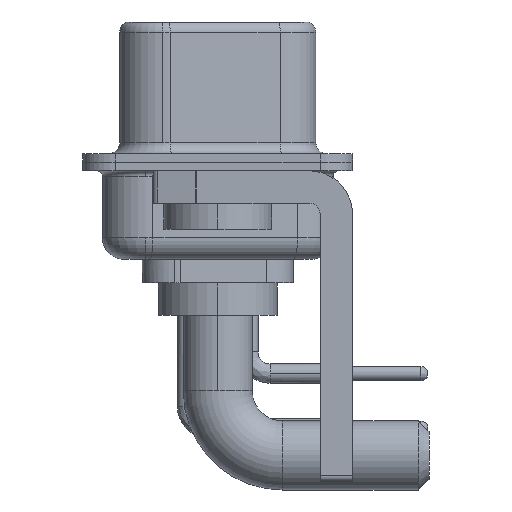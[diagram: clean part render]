
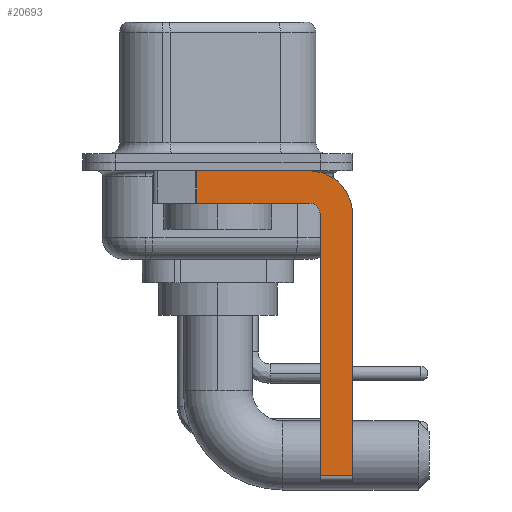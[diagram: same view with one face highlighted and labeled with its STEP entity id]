
A CAD part, left-side view. The second image highlights one B-rep face of the part: STEP entity #20693.
In plain terms, the highlighted planar face has unit normal (-1, 0, 0).
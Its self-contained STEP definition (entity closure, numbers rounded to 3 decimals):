
#100 = CARTESIAN_POINT ( 'NONE',  ( -2.9, -6.25, -2.4 ) ) ;
#116 = VECTOR ( 'NONE', #11203, 1000. ) ;
#220 = CARTESIAN_POINT ( 'NONE',  ( -2.9, 0.978, -1.9 ) ) ;
#757 = AXIS2_PLACEMENT_3D ( 'NONE', #5977, #12629, #12404 ) ;
#1545 = DIRECTION ( 'NONE',  ( 0., 0., -1. ) ) ;
#1931 = ORIENTED_EDGE ( 'NONE', *, *, #10886, .T. ) ;
#2019 = DIRECTION ( 'NONE',  ( 1., 0., 0. ) ) ;
#2078 = ORIENTED_EDGE ( 'NONE', *, *, #13336, .F. ) ;
#2173 = VECTOR ( 'NONE', #6767, 1000. ) ;
#2794 = VERTEX_POINT ( 'NONE', #19829 ) ;
#2855 = CIRCLE ( 'NONE', #9224, 2. ) ;
#3239 = CARTESIAN_POINT ( 'NONE',  ( -2.9, -4.25, -14.55 ) ) ;
#3648 = DIRECTION ( 'NONE',  ( 0., 0., -1. ) ) ;
#3952 = VERTEX_POINT ( 'NONE', #18066 ) ;
#4442 = AXIS2_PLACEMENT_3D ( 'NONE', #19038, #2019, #8884 ) ;
#4966 = VECTOR ( 'NONE', #16935, 1000. ) ;
#5174 = EDGE_CURVE ( 'NONE', #12116, #10707, #8334, .T. ) ;
#5224 = FACE_OUTER_BOUND ( 'NONE', #16651, .T. ) ;
#5962 = VERTEX_POINT ( 'NONE', #18555 ) ;
#5977 = CARTESIAN_POINT ( 'NONE',  ( -2.9, -4.25, -2.4 ) ) ;
#6090 = ORIENTED_EDGE ( 'NONE', *, *, #5174, .F. ) ;
#6448 = LINE ( 'NONE', #220, #4966 ) ;
#6767 = DIRECTION ( 'NONE',  ( 0., -1., 0. ) ) ;
#7126 = ORIENTED_EDGE ( 'NONE', *, *, #14853, .F. ) ;
#7815 = DIRECTION ( 'NONE',  ( 0., 1., 0. ) ) ;
#8334 = LINE ( 'NONE', #16216, #8350 ) ;
#8350 = VECTOR ( 'NONE', #7815, 1000. ) ;
#8528 = LINE ( 'NONE', #100, #18338 ) ;
#8662 = VERTEX_POINT ( 'NONE', #13959 ) ;
#8727 = CARTESIAN_POINT ( 'NONE',  ( -2.9, -4.25, -2.4 ) ) ;
#8881 = ORIENTED_EDGE ( 'NONE', *, *, #19482, .F. ) ;
#8884 = DIRECTION ( 'NONE',  ( 0., 0., -1. ) ) ;
#9224 = AXIS2_PLACEMENT_3D ( 'NONE', #8727, #12156, #1545 ) ;
#9881 = LINE ( 'NONE', #3239, #2173 ) ;
#9993 = CARTESIAN_POINT ( 'NONE',  ( -2.9, -4.75, -14.55 ) ) ;
#10224 = CARTESIAN_POINT ( 'NONE',  ( -2.9, -4.25, -0.4 ) ) ;
#10404 = VERTEX_POINT ( 'NONE', #10224 ) ;
#10707 = VERTEX_POINT ( 'NONE', #17722 ) ;
#10886 = EDGE_CURVE ( 'NONE', #8662, #10707, #6448, .T. ) ;
#10972 = DIRECTION ( 'NONE',  ( 0., 0., 1. ) ) ;
#11089 = EDGE_CURVE ( 'NONE', #17908, #3952, #19578, .T. ) ;
#11203 = DIRECTION ( 'NONE',  ( 0., -1., 0. ) ) ;
#12116 = VERTEX_POINT ( 'NONE', #17726 ) ;
#12156 = DIRECTION ( 'NONE',  ( 1., 0., 0. ) ) ;
#12202 = EDGE_CURVE ( 'NONE', #17908, #5962, #9881, .T. ) ;
#12404 = DIRECTION ( 'NONE',  ( 0., 0., 1. ) ) ;
#12615 = ORIENTED_EDGE ( 'NONE', *, *, #15635, .F. ) ;
#12629 = DIRECTION ( 'NONE',  ( -1., 0., 0. ) ) ;
#12753 = CARTESIAN_POINT ( 'NONE',  ( -2.9, 3., -0.4 ) ) ;
#13078 = ORIENTED_EDGE ( 'NONE', *, *, #11089, .F. ) ;
#13336 = EDGE_CURVE ( 'NONE', #2794, #5962, #8528, .T. ) ;
#13959 = CARTESIAN_POINT ( 'NONE',  ( -2.9, 0.978, -0.4 ) ) ;
#14186 = LINE ( 'NONE', #12753, #116 ) ;
#14853 = EDGE_CURVE ( 'NONE', #10404, #2794, #2855, .T. ) ;
#15635 = EDGE_CURVE ( 'NONE', #3952, #12116, #21607, .T. ) ;
#16216 = CARTESIAN_POINT ( 'NONE',  ( -2.9, -4.25, -1.9 ) ) ;
#16651 = EDGE_LOOP ( 'NONE', ( #8881, #1931, #6090, #12615, #13078, #17465, #2078, #7126 ) ) ;
#16935 = DIRECTION ( 'NONE',  ( 0., 0., -1. ) ) ;
#17378 = PLANE ( 'NONE',  #4442 ) ;
#17465 = ORIENTED_EDGE ( 'NONE', *, *, #12202, .T. ) ;
#17476 = CARTESIAN_POINT ( 'NONE',  ( -2.9, -4.75, -14.8 ) ) ;
#17722 = CARTESIAN_POINT ( 'NONE',  ( -2.9, 0.978, -1.9 ) ) ;
#17726 = CARTESIAN_POINT ( 'NONE',  ( -2.9, -4.25, -1.9 ) ) ;
#17908 = VERTEX_POINT ( 'NONE', #9993 ) ;
#18066 = CARTESIAN_POINT ( 'NONE',  ( -2.9, -4.75, -2.4 ) ) ;
#18338 = VECTOR ( 'NONE', #3648, 1000. ) ;
#18369 = VECTOR ( 'NONE', #10972, 1000. ) ;
#18555 = CARTESIAN_POINT ( 'NONE',  ( -2.9, -6.25, -14.55 ) ) ;
#19038 = CARTESIAN_POINT ( 'NONE',  ( -2.9, -4.25, -2.4 ) ) ;
#19482 = EDGE_CURVE ( 'NONE', #8662, #10404, #14186, .T. ) ;
#19578 = LINE ( 'NONE', #17476, #18369 ) ;
#19829 = CARTESIAN_POINT ( 'NONE',  ( -2.9, -6.25, -2.4 ) ) ;
#20693 = ADVANCED_FACE ( 'NONE', ( #5224 ), #17378, .F. ) ;
#21607 = CIRCLE ( 'NONE', #757, 0.5 ) ;
